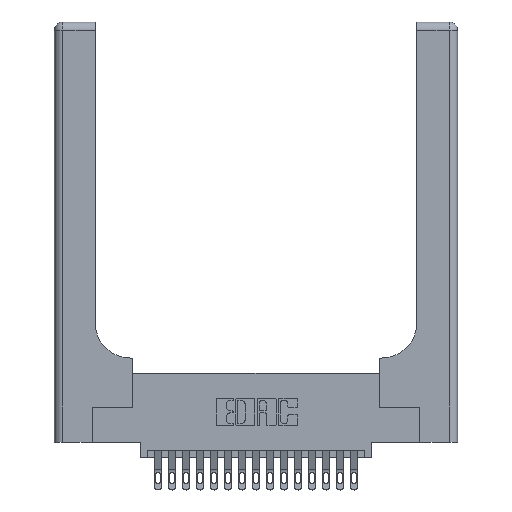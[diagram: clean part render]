
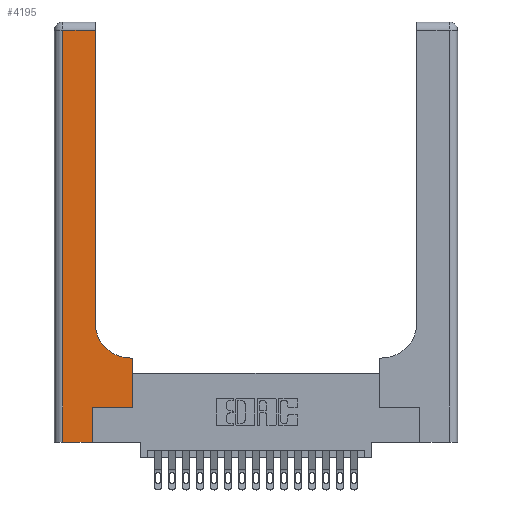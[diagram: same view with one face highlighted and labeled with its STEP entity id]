
A CAD part, top view. The second image highlights one B-rep face of the part: STEP entity #4195.
In plain terms, the highlighted planar face has unit normal (0, 0, 1).
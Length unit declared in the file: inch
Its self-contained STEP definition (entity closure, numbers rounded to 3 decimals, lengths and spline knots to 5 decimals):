
#150 = CARTESIAN_POINT ( 'NONE',  ( 0.06, 0., 0.37 ) ) ;
#227 = ORIENTED_EDGE ( 'NONE', *, *, #17055, .T. ) ;
#618 = DIRECTION ( 'NONE',  ( 0., 1., 0. ) ) ;
#655 = VERTEX_POINT ( 'NONE', #7615 ) ;
#951 = EDGE_CURVE ( 'NONE', #12934, #11187, #12096, .T. ) ;
#1130 = DIRECTION ( 'NONE',  ( 1., 0., 0. ) ) ;
#1161 = DIRECTION ( 'NONE',  ( -1., 0., 0. ) ) ;
#1834 = ORIENTED_EDGE ( 'NONE', *, *, #11685, .T. ) ;
#1947 = DIRECTION ( 'NONE',  ( 1., 0., 0. ) ) ;
#2195 = CARTESIAN_POINT ( 'NONE',  ( 0.269, 0.25, 0.37 ) ) ;
#2622 = DIRECTION ( 'NONE',  ( 0., -1., 0. ) ) ;
#2655 = LINE ( 'NONE', #14221, #15353 ) ;
#2735 = CARTESIAN_POINT ( 'NONE',  ( 0.5415, 0.6, 0.37 ) ) ;
#3138 = VECTOR ( 'NONE', #1161, 39.37008 ) ;
#3249 = VECTOR ( 'NONE', #1947, 39.37008 ) ;
#3603 = DIRECTION ( 'NONE',  ( -1., 0., 0. ) ) ;
#4195 = ADVANCED_FACE ( 'NONE', ( #13661 ), #20532, .F. ) ;
#4430 = CARTESIAN_POINT ( 'NONE',  ( 0.5415, 0.85, 0.37 ) ) ;
#4511 = CARTESIAN_POINT ( 'NONE',  ( 0., 3., 0.37 ) ) ;
#4745 = LINE ( 'NONE', #9542, #3138 ) ;
#5409 = VERTEX_POINT ( 'NONE', #2735 ) ;
#6107 = DIRECTION ( 'NONE',  ( 1., 0., 0. ) ) ;
#6184 = DIRECTION ( 'NONE',  ( 0., 0., -1. ) ) ;
#6481 = VERTEX_POINT ( 'NONE', #9221 ) ;
#6520 = EDGE_CURVE ( 'NONE', #8992, #15523, #2655, .T. ) ;
#7415 = EDGE_CURVE ( 'NONE', #5409, #19648, #16751, .T. ) ;
#7518 = VECTOR ( 'NONE', #3603, 39.37008 ) ;
#7615 = CARTESIAN_POINT ( 'NONE',  ( 0.269, 0., 0.37 ) ) ;
#8100 = VECTOR ( 'NONE', #10860, 39.37008 ) ;
#8306 = CARTESIAN_POINT ( 'NONE',  ( 0.06, 2.94, 0.37 ) ) ;
#8643 = CARTESIAN_POINT ( 'NONE',  ( 0.2915, 0.6, 0.37 ) ) ;
#8682 = ORIENTED_EDGE ( 'NONE', *, *, #16792, .T. ) ;
#8992 = VERTEX_POINT ( 'NONE', #8306 ) ;
#9142 = VECTOR ( 'NONE', #618, 39.37008 ) ;
#9221 = CARTESIAN_POINT ( 'NONE',  ( 0.5585, 0.6, 0.37 ) ) ;
#9242 = CARTESIAN_POINT ( 'NONE',  ( 0.269, 0., 0.37 ) ) ;
#9457 = EDGE_CURVE ( 'NONE', #15523, #655, #15730, .T. ) ;
#9542 = CARTESIAN_POINT ( 'NONE',  ( 0., 2.94, 0.37 ) ) ;
#10860 = DIRECTION ( 'NONE',  ( 0., 1., 0. ) ) ;
#10870 = VECTOR ( 'NONE', #1130, 39.37008 ) ;
#10939 = CARTESIAN_POINT ( 'NONE',  ( 0.2915, 2.94, 0.37 ) ) ;
#10973 = VECTOR ( 'NONE', #20919, 39.37008 ) ;
#11187 = VERTEX_POINT ( 'NONE', #18660 ) ;
#11209 = AXIS2_PLACEMENT_3D ( 'NONE', #4430, #15926, #6107 ) ;
#11357 = LINE ( 'NONE', #8643, #7518 ) ;
#11685 = EDGE_CURVE ( 'NONE', #6481, #5409, #11357, .T. ) ;
#12096 = LINE ( 'NONE', #2195, #3249 ) ;
#12381 = CARTESIAN_POINT ( 'NONE',  ( 0.2915, 3., 0.37 ) ) ;
#12934 = VERTEX_POINT ( 'NONE', #16596 ) ;
#13661 = FACE_OUTER_BOUND ( 'NONE', #19875, .T. ) ;
#14221 = CARTESIAN_POINT ( 'NONE',  ( 0.06, 3., 0.37 ) ) ;
#14305 = ORIENTED_EDGE ( 'NONE', *, *, #16759, .T. ) ;
#14442 = CARTESIAN_POINT ( 'NONE',  ( 0., 0., 0.37 ) ) ;
#14806 = ORIENTED_EDGE ( 'NONE', *, *, #16405, .T. ) ;
#14918 = VERTEX_POINT ( 'NONE', #10939 ) ;
#15107 = CARTESIAN_POINT ( 'NONE',  ( 0.2915, 0.85, 0.37 ) ) ;
#15330 = LINE ( 'NONE', #19392, #10973 ) ;
#15353 = VECTOR ( 'NONE', #2622, 39.37008 ) ;
#15523 = VERTEX_POINT ( 'NONE', #150 ) ;
#15730 = LINE ( 'NONE', #14442, #10870 ) ;
#15926 = DIRECTION ( 'NONE',  ( 0., 0., -1. ) ) ;
#16292 = ORIENTED_EDGE ( 'NONE', *, *, #6520, .T. ) ;
#16405 = EDGE_CURVE ( 'NONE', #14918, #8992, #4745, .T. ) ;
#16596 = CARTESIAN_POINT ( 'NONE',  ( 0.269, 0.25, 0.37 ) ) ;
#16751 = CIRCLE ( 'NONE', #11209, 0.25 ) ;
#16759 = EDGE_CURVE ( 'NONE', #19648, #14918, #17669, .T. ) ;
#16765 = ORIENTED_EDGE ( 'NONE', *, *, #9457, .T. ) ;
#16792 = EDGE_CURVE ( 'NONE', #655, #12934, #17202, .T. ) ;
#17055 = EDGE_CURVE ( 'NONE', #11187, #6481, #15330, .T. ) ;
#17202 = LINE ( 'NONE', #9242, #8100 ) ;
#17252 = ORIENTED_EDGE ( 'NONE', *, *, #951, .T. ) ;
#17509 = DIRECTION ( 'NONE',  ( -1., 0., 0. ) ) ;
#17669 = LINE ( 'NONE', #12381, #9142 ) ;
#18660 = CARTESIAN_POINT ( 'NONE',  ( 0.5585, 0.25, 0.37 ) ) ;
#19176 = ORIENTED_EDGE ( 'NONE', *, *, #7415, .T. ) ;
#19392 = CARTESIAN_POINT ( 'NONE',  ( 0.5585, 0.25, 0.37 ) ) ;
#19409 = AXIS2_PLACEMENT_3D ( 'NONE', #4511, #6184, #17509 ) ;
#19648 = VERTEX_POINT ( 'NONE', #15107 ) ;
#19875 = EDGE_LOOP ( 'NONE', ( #14305, #14806, #16292, #16765, #8682, #17252, #227, #1834, #19176 ) ) ;
#20532 = PLANE ( 'NONE',  #19409 ) ;
#20919 = DIRECTION ( 'NONE',  ( 0., 1., 0. ) ) ;
